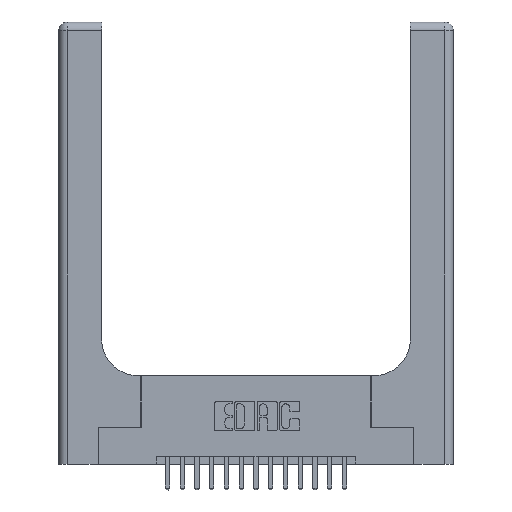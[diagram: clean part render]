
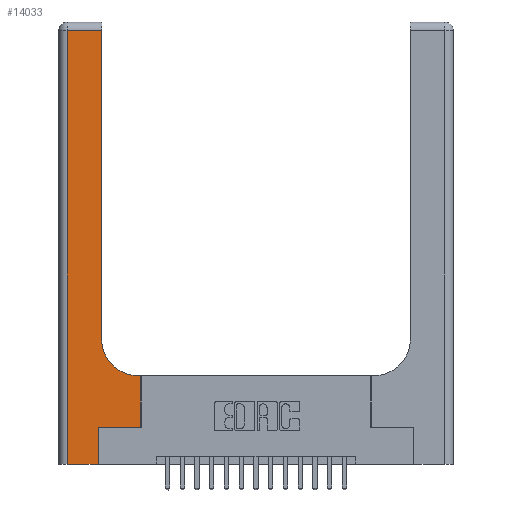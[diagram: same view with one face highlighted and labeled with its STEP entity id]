
A CAD part, top view. The second image highlights one B-rep face of the part: STEP entity #14033.
In plain terms, the highlighted planar face has unit normal (0, 0, 1).
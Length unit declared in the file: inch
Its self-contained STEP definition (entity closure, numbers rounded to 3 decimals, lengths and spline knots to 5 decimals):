
#702 = DIRECTION ( 'NONE',  ( 0., 0., -1. ) ) ;
#1440 = VECTOR ( 'NONE', #13096, 39.37008 ) ;
#1568 = FACE_OUTER_BOUND ( 'NONE', #7883, .T. ) ;
#1596 = CARTESIAN_POINT ( 'NONE',  ( 0.269, 0., 0.37 ) ) ;
#2040 = EDGE_CURVE ( 'NONE', #9907, #4949, #11386, .T. ) ;
#2317 = ORIENTED_EDGE ( 'NONE', *, *, #4868, .T. ) ;
#2901 = CARTESIAN_POINT ( 'NONE',  ( 0.269, 0.25, 0.37 ) ) ;
#3396 = VERTEX_POINT ( 'NONE', #2901 ) ;
#3477 = VERTEX_POINT ( 'NONE', #1596 ) ;
#4789 = DIRECTION ( 'NONE',  ( 0., -1., 0. ) ) ;
#4816 = DIRECTION ( 'NONE',  ( 0., 0., -1. ) ) ;
#4868 = EDGE_CURVE ( 'NONE', #3396, #5112, #10585, .T. ) ;
#4949 = VERTEX_POINT ( 'NONE', #7253 ) ;
#5112 = VERTEX_POINT ( 'NONE', #14180 ) ;
#5836 = LINE ( 'NONE', #6557, #13419 ) ;
#6155 = CARTESIAN_POINT ( 'NONE',  ( 0.269, 0., 0.37 ) ) ;
#6289 = ORIENTED_EDGE ( 'NONE', *, *, #15198, .T. ) ;
#6361 = DIRECTION ( 'NONE',  ( 0., 1., 0. ) ) ;
#6497 = DIRECTION ( 'NONE',  ( -1., 0., 0. ) ) ;
#6557 = CARTESIAN_POINT ( 'NONE',  ( 0.2915, 0.6, 0.37 ) ) ;
#6856 = VERTEX_POINT ( 'NONE', #9590 ) ;
#7009 = VECTOR ( 'NONE', #7679, 39.37008 ) ;
#7127 = LINE ( 'NONE', #15332, #11218 ) ;
#7136 = VERTEX_POINT ( 'NONE', #11786 ) ;
#7253 = CARTESIAN_POINT ( 'NONE',  ( 0.06, 2.94, 0.37 ) ) ;
#7679 = DIRECTION ( 'NONE',  ( 0., 1., 0. ) ) ;
#7883 = EDGE_LOOP ( 'NONE', ( #8334, #19348, #10017, #9711, #6289, #2317, #11106, #13932, #18422 ) ) ;
#8247 = CARTESIAN_POINT ( 'NONE',  ( 0.2915, 3., 0.37 ) ) ;
#8334 = ORIENTED_EDGE ( 'NONE', *, *, #19381, .T. ) ;
#8373 = CARTESIAN_POINT ( 'NONE',  ( 0., 3., 0.37 ) ) ;
#8477 = CARTESIAN_POINT ( 'NONE',  ( 0.06, 0., 0.37 ) ) ;
#8826 = EDGE_CURVE ( 'NONE', #18240, #3477, #11065, .T. ) ;
#8943 = VECTOR ( 'NONE', #4789, 39.37008 ) ;
#9052 = CARTESIAN_POINT ( 'NONE',  ( 0.2915, 2.94, 0.37 ) ) ;
#9590 = CARTESIAN_POINT ( 'NONE',  ( 0.5415, 0.6, 0.37 ) ) ;
#9711 = ORIENTED_EDGE ( 'NONE', *, *, #8826, .T. ) ;
#9813 = AXIS2_PLACEMENT_3D ( 'NONE', #8373, #702, #11467 ) ;
#9907 = VERTEX_POINT ( 'NONE', #9052 ) ;
#10017 = ORIENTED_EDGE ( 'NONE', *, *, #14599, .T. ) ;
#10497 = CIRCLE ( 'NONE', #13218, 0.25 ) ;
#10585 = LINE ( 'NONE', #15974, #1440 ) ;
#10861 = CARTESIAN_POINT ( 'NONE',  ( 0.06, 3., 0.37 ) ) ;
#10916 = VECTOR ( 'NONE', #12076, 39.37008 ) ;
#10999 = EDGE_CURVE ( 'NONE', #5112, #13440, #7127, .T. ) ;
#11065 = LINE ( 'NONE', #18394, #14076 ) ;
#11106 = ORIENTED_EDGE ( 'NONE', *, *, #10999, .T. ) ;
#11198 = LINE ( 'NONE', #8247, #18047 ) ;
#11218 = VECTOR ( 'NONE', #6361, 39.37008 ) ;
#11386 = LINE ( 'NONE', #12304, #10916 ) ;
#11467 = DIRECTION ( 'NONE',  ( -1., 0., 0. ) ) ;
#11786 = CARTESIAN_POINT ( 'NONE',  ( 0.2915, 0.85, 0.37 ) ) ;
#12076 = DIRECTION ( 'NONE',  ( -1., 0., 0. ) ) ;
#12304 = CARTESIAN_POINT ( 'NONE',  ( 0., 2.94, 0.37 ) ) ;
#13096 = DIRECTION ( 'NONE',  ( 1., 0., 0. ) ) ;
#13218 = AXIS2_PLACEMENT_3D ( 'NONE', #13866, #4816, #15294 ) ;
#13419 = VECTOR ( 'NONE', #6497, 39.37008 ) ;
#13440 = VERTEX_POINT ( 'NONE', #18375 ) ;
#13866 = CARTESIAN_POINT ( 'NONE',  ( 0.5415, 0.85, 0.37 ) ) ;
#13932 = ORIENTED_EDGE ( 'NONE', *, *, #16276, .T. ) ;
#14033 = ADVANCED_FACE ( 'NONE', ( #1568 ), #17280, .F. ) ;
#14076 = VECTOR ( 'NONE', #18326, 39.37008 ) ;
#14180 = CARTESIAN_POINT ( 'NONE',  ( 0.5585, 0.25, 0.37 ) ) ;
#14599 = EDGE_CURVE ( 'NONE', #4949, #18240, #17296, .T. ) ;
#15198 = EDGE_CURVE ( 'NONE', #3477, #3396, #19287, .T. ) ;
#15294 = DIRECTION ( 'NONE',  ( 1., 0., 0. ) ) ;
#15332 = CARTESIAN_POINT ( 'NONE',  ( 0.5585, 0.25, 0.37 ) ) ;
#15974 = CARTESIAN_POINT ( 'NONE',  ( 0.269, 0.25, 0.37 ) ) ;
#16276 = EDGE_CURVE ( 'NONE', #13440, #6856, #5836, .T. ) ;
#17280 = PLANE ( 'NONE',  #9813 ) ;
#17296 = LINE ( 'NONE', #10861, #8943 ) ;
#18047 = VECTOR ( 'NONE', #18596, 39.37008 ) ;
#18240 = VERTEX_POINT ( 'NONE', #8477 ) ;
#18326 = DIRECTION ( 'NONE',  ( 1., 0., 0. ) ) ;
#18375 = CARTESIAN_POINT ( 'NONE',  ( 0.5585, 0.6, 0.37 ) ) ;
#18394 = CARTESIAN_POINT ( 'NONE',  ( 0., 0., 0.37 ) ) ;
#18422 = ORIENTED_EDGE ( 'NONE', *, *, #19192, .T. ) ;
#18596 = DIRECTION ( 'NONE',  ( 0., 1., 0. ) ) ;
#19192 = EDGE_CURVE ( 'NONE', #6856, #7136, #10497, .T. ) ;
#19287 = LINE ( 'NONE', #6155, #7009 ) ;
#19348 = ORIENTED_EDGE ( 'NONE', *, *, #2040, .T. ) ;
#19381 = EDGE_CURVE ( 'NONE', #7136, #9907, #11198, .T. ) ;
